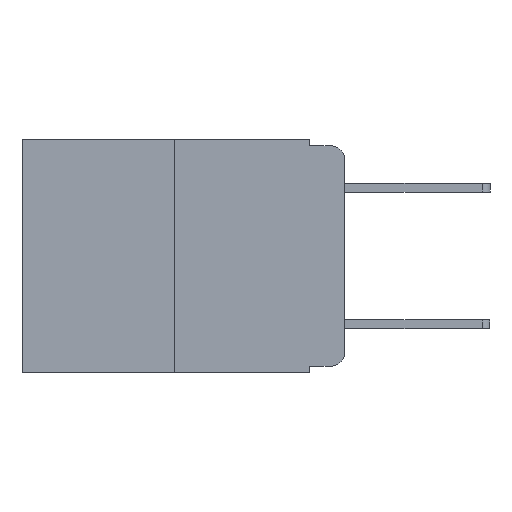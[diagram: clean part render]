
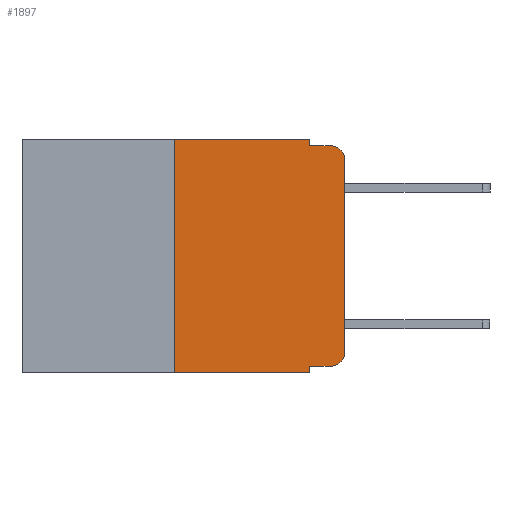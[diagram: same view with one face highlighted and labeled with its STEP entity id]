
A CAD part, left-side view. The second image highlights one B-rep face of the part: STEP entity #1897.
In plain terms, the highlighted planar face has unit normal (-1, 0, 0).
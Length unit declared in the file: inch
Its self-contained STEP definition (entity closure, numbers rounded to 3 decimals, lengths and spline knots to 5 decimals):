
#37 = EDGE_CURVE ( 'NONE', #10398, #10938, #8302, .T. ) ;
#94 = LINE ( 'NONE', #203, #5235 ) ;
#127 = VECTOR ( 'NONE', #3830, 39.37008 ) ;
#203 = CARTESIAN_POINT ( 'NONE',  ( 0., 0.051, -0.01 ) ) ;
#391 = ORIENTED_EDGE ( 'NONE', *, *, #3465, .T. ) ;
#498 = DIRECTION ( 'NONE',  ( 0., 0., -1. ) ) ;
#527 = DIRECTION ( 'NONE',  ( -1., 0., 0. ) ) ;
#565 = EDGE_CURVE ( 'NONE', #9936, #2911, #10373, .T. ) ;
#567 = ORIENTED_EDGE ( 'NONE', *, *, #37, .F. ) ;
#590 = ORIENTED_EDGE ( 'NONE', *, *, #6472, .T. ) ;
#954 = VERTEX_POINT ( 'NONE', #2909 ) ;
#1037 = VECTOR ( 'NONE', #5384, 39.37008 ) ;
#1058 = CARTESIAN_POINT ( 'NONE',  ( 0., 0.473, -0.343 ) ) ;
#1346 = VECTOR ( 'NONE', #4992, 39.37008 ) ;
#1385 = EDGE_CURVE ( 'NONE', #4574, #10398, #3487, .T. ) ;
#1390 = ORIENTED_EDGE ( 'NONE', *, *, #3499, .F. ) ;
#1432 = AXIS2_PLACEMENT_3D ( 'NONE', #3022, #3453, #498 ) ;
#1543 = EDGE_CURVE ( 'NONE', #9936, #4574, #3914, .T. ) ;
#1625 = FACE_OUTER_BOUND ( 'NONE', #6130, .T. ) ;
#1705 = CARTESIAN_POINT ( 'NONE',  ( 0., 0.25, -0.343 ) ) ;
#1875 = LINE ( 'NONE', #2331, #8751 ) ;
#1897 = ADVANCED_FACE ( 'NONE', ( #1625 ), #2584, .F. ) ;
#2331 = CARTESIAN_POINT ( 'NONE',  ( 0., 0.051, 0. ) ) ;
#2584 = PLANE ( 'NONE',  #9162 ) ;
#2595 = DIRECTION ( 'NONE',  ( 0., 0., -1. ) ) ;
#2653 = DIRECTION ( 'NONE',  ( 1., 0., 0. ) ) ;
#2880 = CARTESIAN_POINT ( 'NONE',  ( 0., 0.051, 0. ) ) ;
#2909 = CARTESIAN_POINT ( 'NONE',  ( 0., 0.051, -0.333 ) ) ;
#2911 = VERTEX_POINT ( 'NONE', #8015 ) ;
#3007 = CARTESIAN_POINT ( 'NONE',  ( 0., 0., -0.313 ) ) ;
#3022 = CARTESIAN_POINT ( 'NONE',  ( 0., 0.02, -0.313 ) ) ;
#3090 = ORIENTED_EDGE ( 'NONE', *, *, #10119, .T. ) ;
#3440 = EDGE_CURVE ( 'NONE', #6217, #4557, #3713, .T. ) ;
#3453 = DIRECTION ( 'NONE',  ( -1., 0., 0. ) ) ;
#3465 = EDGE_CURVE ( 'NONE', #4557, #7141, #10311, .T. ) ;
#3487 = LINE ( 'NONE', #9417, #10103 ) ;
#3499 = EDGE_CURVE ( 'NONE', #10938, #7141, #94, .T. ) ;
#3538 = CARTESIAN_POINT ( 'NONE',  ( 0., 0.25, 0. ) ) ;
#3558 = EDGE_CURVE ( 'NONE', #954, #2911, #1875, .T. ) ;
#3713 = LINE ( 'NONE', #10190, #8079 ) ;
#3830 = DIRECTION ( 'NONE',  ( 0., -1., 0. ) ) ;
#3914 = LINE ( 'NONE', #5068, #1346 ) ;
#4403 = AXIS2_PLACEMENT_3D ( 'NONE', #4547, #527, #7870 ) ;
#4468 = CARTESIAN_POINT ( 'NONE',  ( 0., 0., -0.03 ) ) ;
#4547 = CARTESIAN_POINT ( 'NONE',  ( 0., 0.02, -0.03 ) ) ;
#4557 = VERTEX_POINT ( 'NONE', #4468 ) ;
#4574 = VERTEX_POINT ( 'NONE', #3538 ) ;
#4992 = DIRECTION ( 'NONE',  ( 0., 0., 1. ) ) ;
#5035 = DIRECTION ( 'NONE',  ( 0., 0., -1. ) ) ;
#5068 = CARTESIAN_POINT ( 'NONE',  ( 0., 0.25, 0. ) ) ;
#5076 = DIRECTION ( 'NONE',  ( 0., 0., 1. ) ) ;
#5235 = VECTOR ( 'NONE', #6756, 39.37008 ) ;
#5384 = DIRECTION ( 'NONE',  ( 0., 0., -1. ) ) ;
#5531 = LINE ( 'NONE', #8249, #127 ) ;
#5854 = VECTOR ( 'NONE', #6700, 39.37008 ) ;
#6130 = EDGE_LOOP ( 'NONE', ( #7624, #391, #1390, #567, #10406, #6448, #7258, #8067, #3090, #590 ) ) ;
#6217 = VERTEX_POINT ( 'NONE', #3007 ) ;
#6448 = ORIENTED_EDGE ( 'NONE', *, *, #1543, .F. ) ;
#6472 = EDGE_CURVE ( 'NONE', #9074, #6217, #10381, .T. ) ;
#6700 = DIRECTION ( 'NONE',  ( 0., -1., 0. ) ) ;
#6756 = DIRECTION ( 'NONE',  ( 0., -1., 0. ) ) ;
#6893 = CARTESIAN_POINT ( 'NONE',  ( 0., 0.02, -0.333 ) ) ;
#7141 = VERTEX_POINT ( 'NONE', #8473 ) ;
#7258 = ORIENTED_EDGE ( 'NONE', *, *, #565, .T. ) ;
#7295 = CARTESIAN_POINT ( 'NONE',  ( 0., 0.051, -0.01 ) ) ;
#7624 = ORIENTED_EDGE ( 'NONE', *, *, #3440, .T. ) ;
#7870 = DIRECTION ( 'NONE',  ( 0., 0., -1. ) ) ;
#8015 = CARTESIAN_POINT ( 'NONE',  ( 0., 0.051, -0.343 ) ) ;
#8067 = ORIENTED_EDGE ( 'NONE', *, *, #3558, .F. ) ;
#8079 = VECTOR ( 'NONE', #5076, 39.37008 ) ;
#8249 = CARTESIAN_POINT ( 'NONE',  ( 0., 0.051, -0.333 ) ) ;
#8302 = LINE ( 'NONE', #2880, #1037 ) ;
#8473 = CARTESIAN_POINT ( 'NONE',  ( 0., 0.02, -0.01 ) ) ;
#8751 = VECTOR ( 'NONE', #5035, 39.37008 ) ;
#9074 = VERTEX_POINT ( 'NONE', #6893 ) ;
#9162 = AXIS2_PLACEMENT_3D ( 'NONE', #9984, #2653, #2595 ) ;
#9212 = CARTESIAN_POINT ( 'NONE',  ( 0., 0.051, 0. ) ) ;
#9417 = CARTESIAN_POINT ( 'NONE',  ( 0., 0.473, 0. ) ) ;
#9475 = DIRECTION ( 'NONE',  ( 0., -1., 0. ) ) ;
#9936 = VERTEX_POINT ( 'NONE', #1705 ) ;
#9984 = CARTESIAN_POINT ( 'NONE',  ( 0., 0.473, 0. ) ) ;
#10103 = VECTOR ( 'NONE', #9475, 39.37008 ) ;
#10119 = EDGE_CURVE ( 'NONE', #954, #9074, #5531, .T. ) ;
#10190 = CARTESIAN_POINT ( 'NONE',  ( 0., 0., 0. ) ) ;
#10311 = CIRCLE ( 'NONE', #4403, 0.02 ) ;
#10373 = LINE ( 'NONE', #1058, #5854 ) ;
#10381 = CIRCLE ( 'NONE', #1432, 0.02 ) ;
#10398 = VERTEX_POINT ( 'NONE', #9212 ) ;
#10406 = ORIENTED_EDGE ( 'NONE', *, *, #1385, .F. ) ;
#10938 = VERTEX_POINT ( 'NONE', #7295 ) ;
